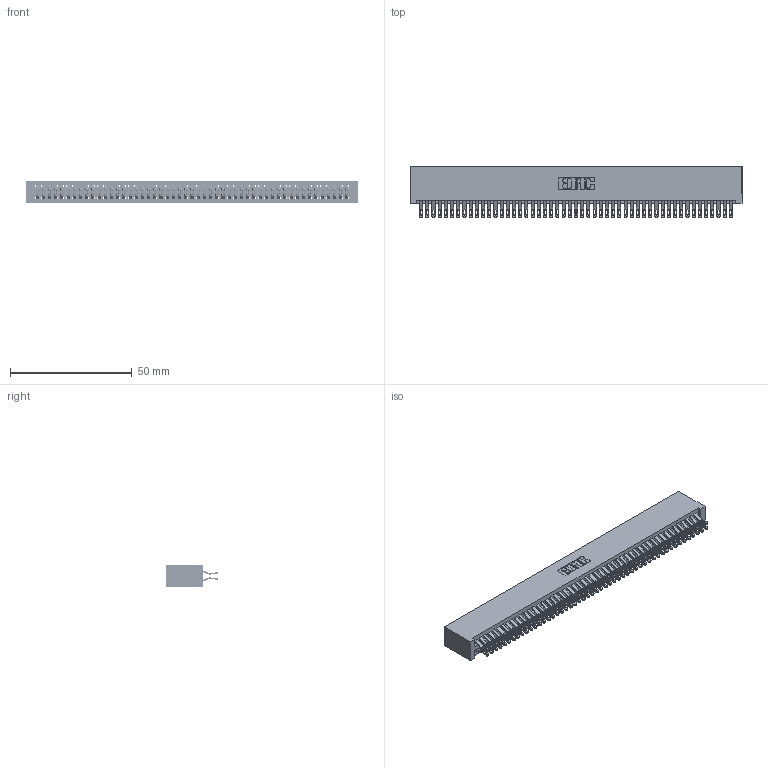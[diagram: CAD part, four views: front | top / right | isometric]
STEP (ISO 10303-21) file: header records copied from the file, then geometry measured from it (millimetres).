
FILE_DESCRIPTION (( 'STEP AP203' ), '1' );
FILE_NAME ('395-102-555-201.STEP', '2019-10-26T18:48:53', ( '' ), ( '' ), 'SwSTEP 2.0', 'SolidWorks 2016', '' );
FILE_SCHEMA (( 'CONFIG_CONTROL_DESIGN' ));
Length unit declared in the file: inch
Products named in the file (3): 345 Part_No Mounting Lugs; 345-292-001_555 Tail; 395-102-555-201
Assembly tree (103 placements, depth 2):
  395-102-555-201
    345 Part_No Mounting Lugs
    345-292-001_555 Tail  x102
Bounding box: 136.14 x 21.13 x 9.4 mm (x, y, z)
Volume: 14220.5 mm3; surface area: 22526.8 mm2
Topology: 103 solids, 103 shells, 5830 faces, 18371 edges, 12246 vertices
Faces by surface type: plane 3238, cylinder 2592
Entity records: 38853 total; most frequent: CARTESIAN_POINT 6538, ORIENTED_EDGE 6442, DIRECTION 5717, EDGE_CURVE 3221, VECTOR 2873, LINE 2873, VERTEX_POINT 2146, AXIS2_PLACEMENT_3D 1422
